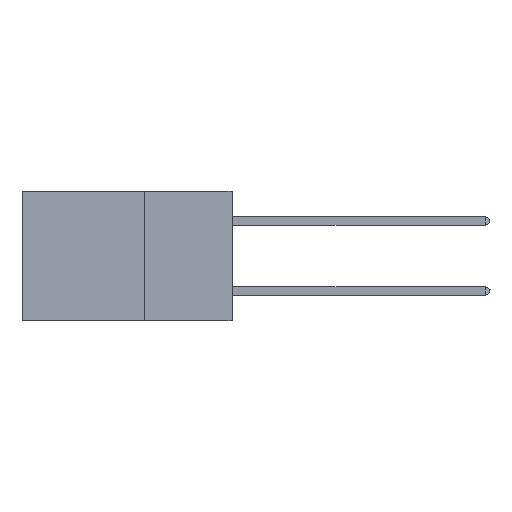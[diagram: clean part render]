
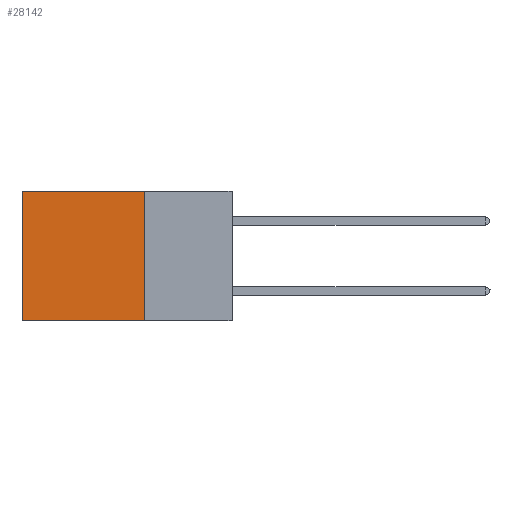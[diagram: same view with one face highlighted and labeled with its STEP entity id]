
A CAD part, left-side view. The second image highlights one B-rep face of the part: STEP entity #28142.
In plain terms, the highlighted planar face has unit normal (-1, 0, 0).
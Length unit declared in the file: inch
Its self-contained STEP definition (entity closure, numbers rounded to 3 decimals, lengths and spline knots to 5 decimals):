
#86 = EDGE_CURVE ( 'NONE', #16084, #8797, #14284, .T. ) ;
#282 = CARTESIAN_POINT ( 'NONE',  ( 0.2875, 0.25, 0. ) ) ;
#2585 = EDGE_LOOP ( 'NONE', ( #8657, #27849, #28158, #29431 ) ) ;
#3625 = CARTESIAN_POINT ( 'NONE',  ( 0.2875, 0.6, -0.37 ) ) ;
#3874 = VECTOR ( 'NONE', #5501, 39.37008 ) ;
#3908 = CARTESIAN_POINT ( 'NONE',  ( 0.2875, 0.25, 0. ) ) ;
#5179 = LINE ( 'NONE', #10265, #3874 ) ;
#5293 = VERTEX_POINT ( 'NONE', #21407 ) ;
#5501 = DIRECTION ( 'NONE',  ( 0., 1., 0. ) ) ;
#6916 = DIRECTION ( 'NONE',  ( 1., 0., 0. ) ) ;
#7317 = CARTESIAN_POINT ( 'NONE',  ( 0.2875, 0.6, 0. ) ) ;
#8112 = DIRECTION ( 'NONE',  ( 0., 0., -1. ) ) ;
#8657 = ORIENTED_EDGE ( 'NONE', *, *, #19903, .T. ) ;
#8676 = FACE_OUTER_BOUND ( 'NONE', #2585, .T. ) ;
#8797 = VERTEX_POINT ( 'NONE', #3625 ) ;
#10265 = CARTESIAN_POINT ( 'NONE',  ( 0.2875, 0.25, 0. ) ) ;
#11340 = EDGE_CURVE ( 'NONE', #20267, #5293, #5179, .T. ) ;
#11366 = PLANE ( 'NONE',  #24401 ) ;
#14127 = DIRECTION ( 'NONE',  ( 0., 1., 0. ) ) ;
#14284 = LINE ( 'NONE', #26450, #24774 ) ;
#14438 = VECTOR ( 'NONE', #8112, 39.37008 ) ;
#15077 = CARTESIAN_POINT ( 'NONE',  ( 0.2875, 0.25, 0. ) ) ;
#15529 = LINE ( 'NONE', #15077, #14438 ) ;
#16084 = VERTEX_POINT ( 'NONE', #20578 ) ;
#16563 = DIRECTION ( 'NONE',  ( 0., 0., -1. ) ) ;
#19903 = EDGE_CURVE ( 'NONE', #5293, #8797, #22347, .T. ) ;
#19977 = DIRECTION ( 'NONE',  ( 0., 0., -1. ) ) ;
#20267 = VERTEX_POINT ( 'NONE', #282 ) ;
#20578 = CARTESIAN_POINT ( 'NONE',  ( 0.2875, 0.25, -0.37 ) ) ;
#21407 = CARTESIAN_POINT ( 'NONE',  ( 0.2875, 0.6, 0. ) ) ;
#22347 = LINE ( 'NONE', #7317, #23904 ) ;
#23904 = VECTOR ( 'NONE', #19977, 39.37008 ) ;
#24401 = AXIS2_PLACEMENT_3D ( 'NONE', #3908, #6916, #16563 ) ;
#24774 = VECTOR ( 'NONE', #14127, 39.37008 ) ;
#26450 = CARTESIAN_POINT ( 'NONE',  ( 0.2875, 0.25, -0.37 ) ) ;
#27849 = ORIENTED_EDGE ( 'NONE', *, *, #86, .F. ) ;
#28142 = ADVANCED_FACE ( 'NONE', ( #8676 ), #11366, .F. ) ;
#28158 = ORIENTED_EDGE ( 'NONE', *, *, #30729, .F. ) ;
#29431 = ORIENTED_EDGE ( 'NONE', *, *, #11340, .T. ) ;
#30729 = EDGE_CURVE ( 'NONE', #20267, #16084, #15529, .T. ) ;
